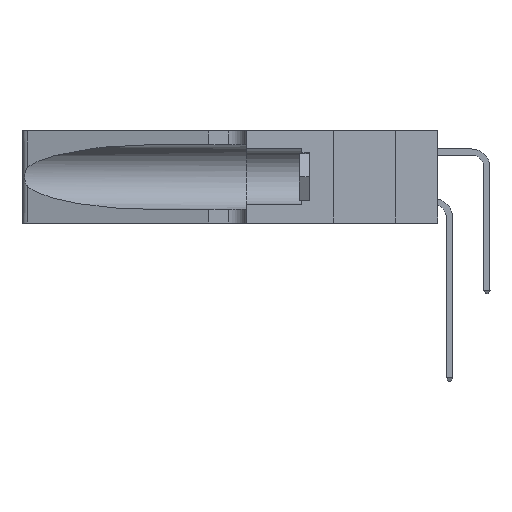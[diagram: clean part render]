
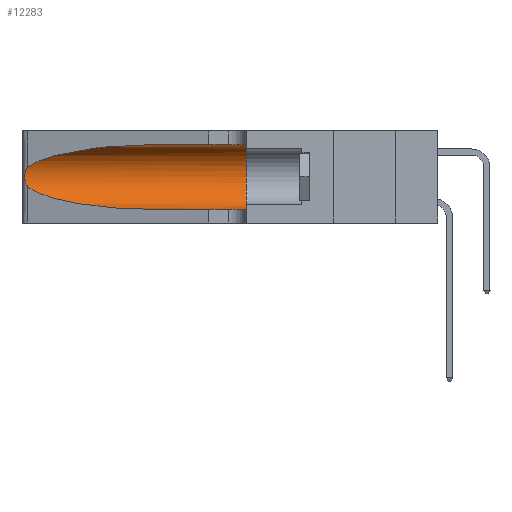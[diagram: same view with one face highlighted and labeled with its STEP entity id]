
A CAD part, left-side view. The second image highlights one B-rep face of the part: STEP entity #12283.
In plain terms, the highlighted cylindrical face has radius 3.308 mm (diameter 6.617 mm), a partial arc.
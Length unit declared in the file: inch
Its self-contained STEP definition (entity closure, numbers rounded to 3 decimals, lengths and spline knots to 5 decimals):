
#121 = ORIENTED_EDGE ( 'NONE', *, *, #5644, .T. ) ;
#276 = VERTEX_POINT ( 'NONE', #2392 ) ;
#335 = ORIENTED_EDGE ( 'NONE', *, *, #2214, .T. ) ;
#928 = CARTESIAN_POINT ( 'NONE',  ( 0.26018, 1.23835, 0.19895 ) ) ;
#1039 = ORIENTED_EDGE ( 'NONE', *, *, #7273, .T. ) ;
#1244 = CARTESIAN_POINT ( 'NONE',  ( 0.1305, 0.72297, 0.31525 ) ) ;
#1277 = CARTESIAN_POINT ( 'NONE',  ( 0.1305, 0.35, 0.31525 ) ) ;
#1502 = ORIENTED_EDGE ( 'NONE', *, *, #6783, .T. ) ;
#1672 = CARTESIAN_POINT ( 'NONE',  ( 0.1305, 0.35, 0.05475 ) ) ;
#1766 = DIRECTION ( 'NONE',  ( 0., -1., 0. ) ) ;
#2214 = EDGE_CURVE ( 'NONE', #10420, #7581, #18523, .T. ) ;
#2392 = CARTESIAN_POINT ( 'NONE',  ( 0.25487, 1.22718, 0.14631 ) ) ;
#2693 = CARTESIAN_POINT ( 'NONE',  ( 0.26075, 1.23896, 0.178 ) ) ;
#2943 = CYLINDRICAL_SURFACE ( 'NONE', #21565, 0.13025 ) ;
#3344 = EDGE_LOOP ( 'NONE', ( #335, #121, #1502, #1039, #11869, #14140 ) ) ;
#3667 = CARTESIAN_POINT ( 'NONE',  ( 0.2373, 1.15595, 0.08982 ) ) ;
#4087 = CARTESIAN_POINT ( 'NONE',  ( 0.25487, 1.22718, 0.22369 ) ) ;
#4262 = DIRECTION ( 'NONE',  ( 0., -1., 0. ) ) ;
#4330 = CARTESIAN_POINT ( 'NONE',  ( 0.18966, 0.96281, 0.31525 ) ) ;
#4456 = CARTESIAN_POINT ( 'NONE',  ( 0.25856, 1.23593, 0.16098 ) ) ;
#5269 = EDGE_CURVE ( 'NONE', #16572, #14710, #11796, .T. ) ;
#5392 = CARTESIAN_POINT ( 'NONE',  ( 0.18966, 0.96281, 0.05475 ) ) ;
#5644 = EDGE_CURVE ( 'NONE', #7581, #276, #20365, .T. ) ;
#6006 = CARTESIAN_POINT ( 'NONE',  ( 0.1305, 1.61858, 0.185 ) ) ;
#6138 = CARTESIAN_POINT ( 'NONE',  ( 0.25555, 1.22994, 0.2215 ) ) ;
#6210 = CARTESIAN_POINT ( 'NONE',  ( 0.25639, 1.23186, 0.15144 ) ) ;
#6244 = VECTOR ( 'NONE', #1766, 39.37008 ) ;
#6783 = EDGE_CURVE ( 'NONE', #276, #17778, #12702, .T. ) ;
#6829 = CARTESIAN_POINT ( 'NONE',  ( 0.1305, 0.72297, 0.31525 ) ) ;
#6935 = CARTESIAN_POINT ( 'NONE',  ( 0.1305, 1.61858, 0.31525 ) ) ;
#7273 = EDGE_CURVE ( 'NONE', #17778, #14710, #16362, .T. ) ;
#7581 = VERTEX_POINT ( 'NONE', #4087 ) ;
#7924 = CARTESIAN_POINT ( 'NONE',  ( 0.25487, 1.22718, 0.14631 ) ) ;
#8581 = EDGE_CURVE ( 'NONE', #10420, #16572, #10775, .T. ) ;
#9581 = CARTESIAN_POINT ( 'NONE',  ( 0.25639, 1.23184, 0.21858 ) ) ;
#10254 = DIRECTION ( 'NONE',  ( 0., 1., 0. ) ) ;
#10420 = VERTEX_POINT ( 'NONE', #6829 ) ;
#10775 = LINE ( 'NONE', #6935, #6244 ) ;
#11282 = CARTESIAN_POINT ( 'NONE',  ( 0.25854, 1.2359, 0.20912 ) ) ;
#11796 = CIRCLE ( 'NONE', #17047, 0.13025 ) ;
#11869 = ORIENTED_EDGE ( 'NONE', *, *, #5269, .F. ) ;
#11999 = CARTESIAN_POINT ( 'NONE',  ( 0.2373, 1.15595, 0.28018 ) ) ;
#12283 = ADVANCED_FACE ( 'NONE', ( #21418 ), #2943, .F. ) ;
#12702 =( BOUNDED_CURVE ( )  B_SPLINE_CURVE ( 3, ( #15613, #3667, #5392, #17239 ),
 .UNSPECIFIED., .F., .T. ) 
 B_SPLINE_CURVE_WITH_KNOTS ( ( 4, 4 ),
 ( 3.44316, 4.71239 ),
 .UNSPECIFIED. ) 
 CURVE ( )  GEOMETRIC_REPRESENTATION_ITEM ( )  RATIONAL_B_SPLINE_CURVE ( ( 1., 0.87, 0.87, 1. ) ) 
 REPRESENTATION_ITEM ( '' )  );
#12818 = DIRECTION ( 'NONE',  ( 0., 0., -1. ) ) ;
#13003 = CARTESIAN_POINT ( 'NONE',  ( 0.26075, 1.23896, 0.19203 ) ) ;
#14140 = ORIENTED_EDGE ( 'NONE', *, *, #8581, .F. ) ;
#14491 = CARTESIAN_POINT ( 'NONE',  ( 0.1305, 0.72297, 0.05475 ) ) ;
#14692 = CARTESIAN_POINT ( 'NONE',  ( 0.26017, 1.23833, 0.17102 ) ) ;
#14710 = VERTEX_POINT ( 'NONE', #1672 ) ;
#15613 = CARTESIAN_POINT ( 'NONE',  ( 0.25487, 1.22718, 0.14631 ) ) ;
#15850 = VECTOR ( 'NONE', #20079, 39.37008 ) ;
#16340 = CARTESIAN_POINT ( 'NONE',  ( 0.25789, 1.23486, 0.15765 ) ) ;
#16362 = LINE ( 'NONE', #16858, #15850 ) ;
#16572 = VERTEX_POINT ( 'NONE', #1277 ) ;
#16858 = CARTESIAN_POINT ( 'NONE',  ( 0.1305, 1.61858, 0.05475 ) ) ;
#17047 = AXIS2_PLACEMENT_3D ( 'NONE', #20213, #10254, #21884 ) ;
#17239 = CARTESIAN_POINT ( 'NONE',  ( 0.1305, 0.72297, 0.05475 ) ) ;
#17778 = VERTEX_POINT ( 'NONE', #14491 ) ;
#17913 = CARTESIAN_POINT ( 'NONE',  ( 0.25487, 1.22718, 0.22369 ) ) ;
#17980 = CARTESIAN_POINT ( 'NONE',  ( 0.25555, 1.22993, 0.14849 ) ) ;
#18523 =( BOUNDED_CURVE ( )  B_SPLINE_CURVE ( 3, ( #1244, #4330, #11999, #18933 ),
 .UNSPECIFIED., .F., .F. ) 
 B_SPLINE_CURVE_WITH_KNOTS ( ( 4, 4 ),
 ( 1.5708, 2.84003 ),
 .UNSPECIFIED. ) 
 CURVE ( )  GEOMETRIC_REPRESENTATION_ITEM ( )  RATIONAL_B_SPLINE_CURVE ( ( 1., 0.87, 0.87, 1. ) ) 
 REPRESENTATION_ITEM ( '' )  );
#18933 = CARTESIAN_POINT ( 'NONE',  ( 0.25487, 1.22718, 0.22369 ) ) ;
#20079 = DIRECTION ( 'NONE',  ( 0., -1., 0. ) ) ;
#20213 = CARTESIAN_POINT ( 'NONE',  ( 0.1305, 0.35, 0.185 ) ) ;
#20365 = B_SPLINE_CURVE_WITH_KNOTS ( 'NONE', 3,
 ( #17913, #6138, #9581, #21222, #11282, #928, #13003, #2693, #14692, #4456, #16340, #6210, #17980, #7924 ),
 .UNSPECIFIED., .F., .F.,
 ( 4, 2, 2, 2, 2, 2, 4 ),
 ( 0., 0.00027, 0.00053, 0.00107, 0.0016, 0.00187, 0.00214 ),
 .UNSPECIFIED. ) ;
#21222 = CARTESIAN_POINT ( 'NONE',  ( 0.25787, 1.23484, 0.2124 ) ) ;
#21418 = FACE_OUTER_BOUND ( 'NONE', #3344, .T. ) ;
#21565 = AXIS2_PLACEMENT_3D ( 'NONE', #6006, #4262, #12818 ) ;
#21884 = DIRECTION ( 'NONE',  ( 0., 0., 1. ) ) ;
